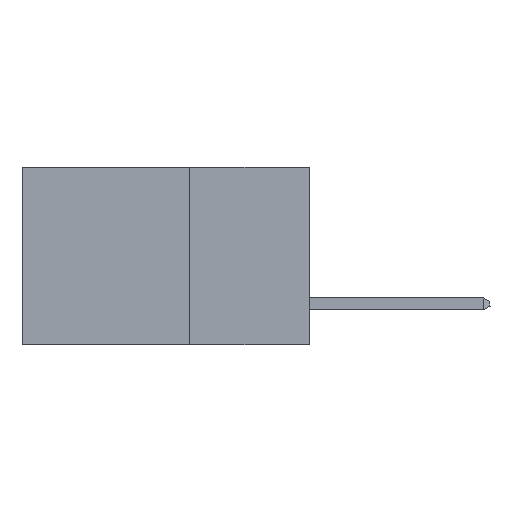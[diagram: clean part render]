
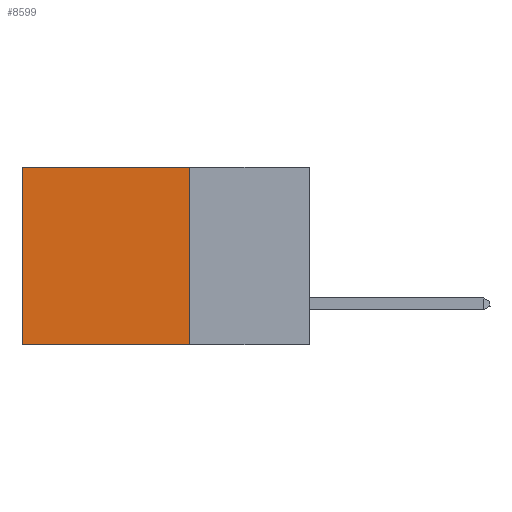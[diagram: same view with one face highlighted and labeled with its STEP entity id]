
A CAD part, left-side view. The second image highlights one B-rep face of the part: STEP entity #8599.
In plain terms, the highlighted planar face has unit normal (-1, 0, 0).
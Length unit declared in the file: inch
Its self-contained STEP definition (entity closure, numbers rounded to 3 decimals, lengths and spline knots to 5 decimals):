
#1121 = CARTESIAN_POINT ( 'NONE',  ( 0.2875, 0.25, -0.37 ) ) ;
#2203 = VECTOR ( 'NONE', #22384, 39.37008 ) ;
#2993 = CARTESIAN_POINT ( 'NONE',  ( 0.2875, 0.25, 0. ) ) ;
#4234 = DIRECTION ( 'NONE',  ( 0., 1., 0. ) ) ;
#5444 = EDGE_LOOP ( 'NONE', ( #6131, #23732, #10032, #27145 ) ) ;
#6131 = ORIENTED_EDGE ( 'NONE', *, *, #21340, .T. ) ;
#7290 = VECTOR ( 'NONE', #4234, 39.37008 ) ;
#7663 = DIRECTION ( 'NONE',  ( 0., 0., -1. ) ) ;
#8599 = ADVANCED_FACE ( 'NONE', ( #9869 ), #15240, .F. ) ;
#9202 = LINE ( 'NONE', #31183, #7290 ) ;
#9869 = FACE_OUTER_BOUND ( 'NONE', #5444, .T. ) ;
#10032 = ORIENTED_EDGE ( 'NONE', *, *, #11885, .F. ) ;
#11144 = VECTOR ( 'NONE', #31086, 39.37008 ) ;
#11885 = EDGE_CURVE ( 'NONE', #26155, #21972, #26114, .T. ) ;
#12883 = CARTESIAN_POINT ( 'NONE',  ( 0.2875, 0.6, 0. ) ) ;
#13617 = EDGE_CURVE ( 'NONE', #21972, #29583, #9202, .T. ) ;
#15158 = LINE ( 'NONE', #29403, #19380 ) ;
#15240 = PLANE ( 'NONE',  #22246 ) ;
#15346 = DIRECTION ( 'NONE',  ( 1., 0., 0. ) ) ;
#15934 = LINE ( 'NONE', #12883, #2203 ) ;
#17611 = VERTEX_POINT ( 'NONE', #20281 ) ;
#18354 = CARTESIAN_POINT ( 'NONE',  ( 0.2875, 0.6, -0.37 ) ) ;
#18784 = CARTESIAN_POINT ( 'NONE',  ( 0.2875, 0.25, 0. ) ) ;
#19380 = VECTOR ( 'NONE', #19538, 39.37008 ) ;
#19538 = DIRECTION ( 'NONE',  ( 0., 1., 0. ) ) ;
#20281 = CARTESIAN_POINT ( 'NONE',  ( 0.2875, 0.6, 0. ) ) ;
#21283 = EDGE_CURVE ( 'NONE', #26155, #17611, #15158, .T. ) ;
#21340 = EDGE_CURVE ( 'NONE', #17611, #29583, #15934, .T. ) ;
#21972 = VERTEX_POINT ( 'NONE', #1121 ) ;
#22246 = AXIS2_PLACEMENT_3D ( 'NONE', #2993, #15346, #7663 ) ;
#22384 = DIRECTION ( 'NONE',  ( 0., 0., -1. ) ) ;
#23732 = ORIENTED_EDGE ( 'NONE', *, *, #13617, .F. ) ;
#26114 = LINE ( 'NONE', #18784, #11144 ) ;
#26155 = VERTEX_POINT ( 'NONE', #28168 ) ;
#27145 = ORIENTED_EDGE ( 'NONE', *, *, #21283, .T. ) ;
#28168 = CARTESIAN_POINT ( 'NONE',  ( 0.2875, 0.25, 0. ) ) ;
#29403 = CARTESIAN_POINT ( 'NONE',  ( 0.2875, 0.25, 0. ) ) ;
#29583 = VERTEX_POINT ( 'NONE', #18354 ) ;
#31086 = DIRECTION ( 'NONE',  ( 0., 0., -1. ) ) ;
#31183 = CARTESIAN_POINT ( 'NONE',  ( 0.2875, 0.25, -0.37 ) ) ;
